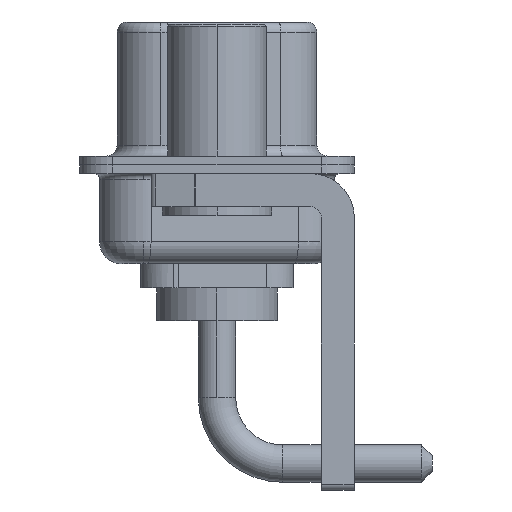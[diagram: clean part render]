
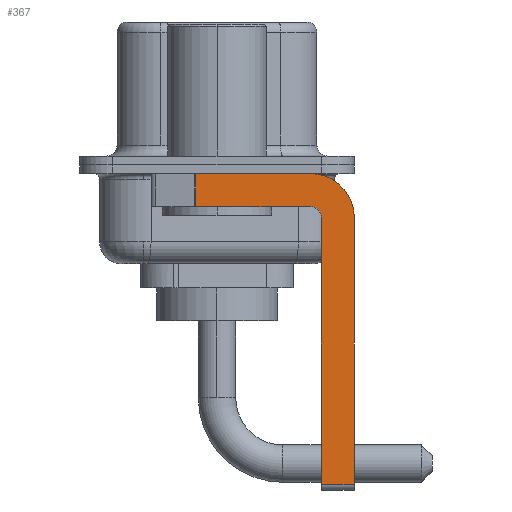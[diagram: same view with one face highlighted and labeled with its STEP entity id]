
A CAD part, left-side view. The second image highlights one B-rep face of the part: STEP entity #367.
In plain terms, the highlighted planar face has unit normal (-1, 0, 0).
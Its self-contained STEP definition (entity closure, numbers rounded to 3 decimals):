
#24 = AXIS2_PLACEMENT_3D ( 'NONE', #11541, #3999, #7656 ) ;
#218 = ORIENTED_EDGE ( 'NONE', *, *, #17624, .T. ) ;
#367 = ADVANCED_FACE ( 'NONE', ( #9037 ), #6002, .F. ) ;
#514 = CARTESIAN_POINT ( 'NONE',  ( -2.9, 0.978, -1.9 ) ) ;
#548 = ORIENTED_EDGE ( 'NONE', *, *, #7496, .F. ) ;
#677 = VECTOR ( 'NONE', #3621, 1000. ) ;
#927 = CIRCLE ( 'NONE', #24, 2. ) ;
#933 = VECTOR ( 'NONE', #2521, 1000. ) ;
#1030 = VECTOR ( 'NONE', #5979, 1000. ) ;
#1033 = DIRECTION ( 'NONE',  ( -1., 0., 0. ) ) ;
#1101 = LINE ( 'NONE', #14189, #933 ) ;
#1224 = CARTESIAN_POINT ( 'NONE',  ( -2.9, -6.25, -2.4 ) ) ;
#1472 = VECTOR ( 'NONE', #14330, 1000. ) ;
#2521 = DIRECTION ( 'NONE',  ( 0., -1., 0. ) ) ;
#2640 = DIRECTION ( 'NONE',  ( 0., 0., 1. ) ) ;
#2814 = EDGE_CURVE ( 'NONE', #10739, #17123, #927, .T. ) ;
#2916 = CARTESIAN_POINT ( 'NONE',  ( -2.9, -4.25, -2.4 ) ) ;
#3322 = EDGE_CURVE ( 'NONE', #9086, #17151, #11513, .T. ) ;
#3470 = DIRECTION ( 'NONE',  ( 1., 0., 0. ) ) ;
#3513 = VERTEX_POINT ( 'NONE', #4421 ) ;
#3621 = DIRECTION ( 'NONE',  ( 0., 0., -1. ) ) ;
#3677 = CARTESIAN_POINT ( 'NONE',  ( -2.9, -4.25, -1.9 ) ) ;
#3826 = CARTESIAN_POINT ( 'NONE',  ( -2.9, -6.25, -2.4 ) ) ;
#3873 = CARTESIAN_POINT ( 'NONE',  ( -2.9, -4.25, -0.4 ) ) ;
#3925 = EDGE_CURVE ( 'NONE', #3513, #9086, #12593, .T. ) ;
#3999 = DIRECTION ( 'NONE',  ( 1., 0., 0. ) ) ;
#4421 = CARTESIAN_POINT ( 'NONE',  ( -2.9, -4.75, -2.4 ) ) ;
#4450 = AXIS2_PLACEMENT_3D ( 'NONE', #2916, #1033, #2640 ) ;
#4827 = CARTESIAN_POINT ( 'NONE',  ( -2.9, -4.75, -14.8 ) ) ;
#5009 = LINE ( 'NONE', #13157, #1030 ) ;
#5886 = ORIENTED_EDGE ( 'NONE', *, *, #3322, .F. ) ;
#5909 = CARTESIAN_POINT ( 'NONE',  ( -2.9, -6.25, -14.55 ) ) ;
#5979 = DIRECTION ( 'NONE',  ( 0., -1., 0. ) ) ;
#6002 = PLANE ( 'NONE',  #17564 ) ;
#6420 = DIRECTION ( 'NONE',  ( 0., 0., 1. ) ) ;
#6458 = EDGE_CURVE ( 'NONE', #14880, #3513, #16319, .T. ) ;
#6702 = EDGE_LOOP ( 'NONE', ( #11147, #12919, #5886, #7823, #14156, #218, #548, #10093 ) ) ;
#6732 = DIRECTION ( 'NONE',  ( 0., 0., -1. ) ) ;
#7496 = EDGE_CURVE ( 'NONE', #17123, #17231, #13517, .T. ) ;
#7605 = CARTESIAN_POINT ( 'NONE',  ( -2.9, -4.25, -2.4 ) ) ;
#7656 = DIRECTION ( 'NONE',  ( 0., 0., -1. ) ) ;
#7823 = ORIENTED_EDGE ( 'NONE', *, *, #3925, .F. ) ;
#9037 = FACE_OUTER_BOUND ( 'NONE', #6702, .T. ) ;
#9086 = VERTEX_POINT ( 'NONE', #3677 ) ;
#9277 = VECTOR ( 'NONE', #6732, 1000. ) ;
#10093 = ORIENTED_EDGE ( 'NONE', *, *, #2814, .F. ) ;
#10739 = VERTEX_POINT ( 'NONE', #3873 ) ;
#11147 = ORIENTED_EDGE ( 'NONE', *, *, #11901, .F. ) ;
#11325 = CARTESIAN_POINT ( 'NONE',  ( -2.9, -4.25, -1.9 ) ) ;
#11501 = CARTESIAN_POINT ( 'NONE',  ( -2.9, 0.978, -0.4 ) ) ;
#11513 = LINE ( 'NONE', #11325, #1472 ) ;
#11541 = CARTESIAN_POINT ( 'NONE',  ( -2.9, -4.25, -2.4 ) ) ;
#11901 = EDGE_CURVE ( 'NONE', #17046, #10739, #1101, .T. ) ;
#12017 = LINE ( 'NONE', #514, #677 ) ;
#12052 = CARTESIAN_POINT ( 'NONE',  ( -2.9, 0.978, -1.9 ) ) ;
#12593 = CIRCLE ( 'NONE', #4450, 0.5 ) ;
#12919 = ORIENTED_EDGE ( 'NONE', *, *, #13219, .T. ) ;
#13157 = CARTESIAN_POINT ( 'NONE',  ( -2.9, -4.25, -14.55 ) ) ;
#13219 = EDGE_CURVE ( 'NONE', #17046, #17151, #12017, .T. ) ;
#13360 = DIRECTION ( 'NONE',  ( 0., 0., -1. ) ) ;
#13517 = LINE ( 'NONE', #3826, #9277 ) ;
#14156 = ORIENTED_EDGE ( 'NONE', *, *, #6458, .F. ) ;
#14189 = CARTESIAN_POINT ( 'NONE',  ( -2.9, 3., -0.4 ) ) ;
#14330 = DIRECTION ( 'NONE',  ( 0., 1., 0. ) ) ;
#14629 = CARTESIAN_POINT ( 'NONE',  ( -2.9, -4.75, -14.55 ) ) ;
#14676 = VECTOR ( 'NONE', #6420, 1000. ) ;
#14880 = VERTEX_POINT ( 'NONE', #14629 ) ;
#16319 = LINE ( 'NONE', #4827, #14676 ) ;
#17046 = VERTEX_POINT ( 'NONE', #11501 ) ;
#17123 = VERTEX_POINT ( 'NONE', #1224 ) ;
#17151 = VERTEX_POINT ( 'NONE', #12052 ) ;
#17231 = VERTEX_POINT ( 'NONE', #5909 ) ;
#17564 = AXIS2_PLACEMENT_3D ( 'NONE', #7605, #3470, #13360 ) ;
#17624 = EDGE_CURVE ( 'NONE', #14880, #17231, #5009, .T. ) ;
